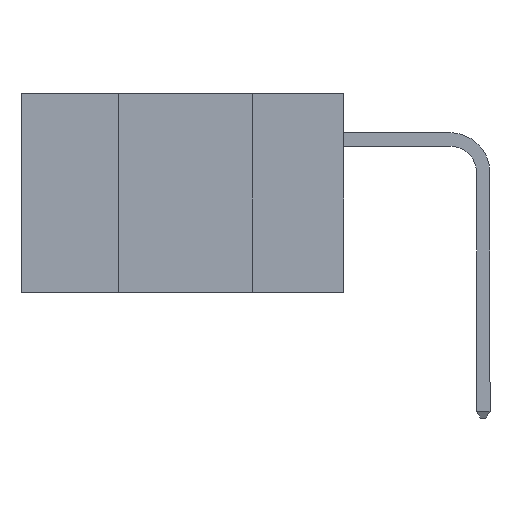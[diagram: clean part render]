
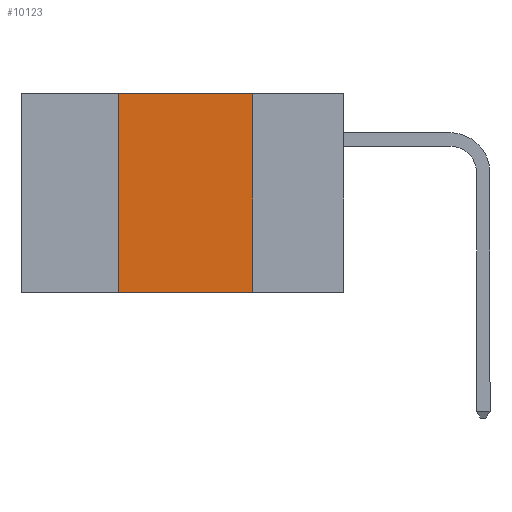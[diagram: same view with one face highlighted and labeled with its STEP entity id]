
A CAD part, left-side view. The second image highlights one B-rep face of the part: STEP entity #10123.
In plain terms, the highlighted planar face has unit normal (-1, 0, 0).
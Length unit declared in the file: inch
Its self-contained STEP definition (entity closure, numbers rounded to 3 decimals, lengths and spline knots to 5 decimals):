
#3 = VECTOR ( 'NONE', #8634, 39.37008 ) ;
#94 = VECTOR ( 'NONE', #7449, 39.37008 ) ;
#901 = CARTESIAN_POINT ( 'NONE',  ( 0., 0.42, -0.37 ) ) ;
#1397 = ORIENTED_EDGE ( 'NONE', *, *, #11086, .F. ) ;
#2379 = FACE_OUTER_BOUND ( 'NONE', #9345, .T. ) ;
#2935 = CARTESIAN_POINT ( 'NONE',  ( 0., 0.17, 0. ) ) ;
#3398 = DIRECTION ( 'NONE',  ( 0., 0., 1. ) ) ;
#3861 = ORIENTED_EDGE ( 'NONE', *, *, #10646, .F. ) ;
#4122 = DIRECTION ( 'NONE',  ( 1., 0., 0. ) ) ;
#6279 = CARTESIAN_POINT ( 'NONE',  ( 0., 0.42, 0. ) ) ;
#6546 = VERTEX_POINT ( 'NONE', #17685 ) ;
#6802 = LINE ( 'NONE', #18522, #3 ) ;
#7359 = VECTOR ( 'NONE', #3398, 39.37008 ) ;
#7449 = DIRECTION ( 'NONE',  ( 0., 0., -1. ) ) ;
#7548 = DIRECTION ( 'NONE',  ( 0., -1., 0. ) ) ;
#7819 = LINE ( 'NONE', #6279, #7359 ) ;
#8634 = DIRECTION ( 'NONE',  ( 0., -1., 0. ) ) ;
#8967 = CARTESIAN_POINT ( 'NONE',  ( 0., 0.6, 0. ) ) ;
#9027 = EDGE_CURVE ( 'NONE', #12057, #12809, #14076, .T. ) ;
#9345 = EDGE_LOOP ( 'NONE', ( #1397, #15475, #3861, #18478 ) ) ;
#9872 = CARTESIAN_POINT ( 'NONE',  ( 0., 0.42, 0. ) ) ;
#9939 = PLANE ( 'NONE',  #12224 ) ;
#10123 = ADVANCED_FACE ( 'NONE', ( #2379 ), #9939, .F. ) ;
#10377 = VECTOR ( 'NONE', #7548, 39.37008 ) ;
#10646 = EDGE_CURVE ( 'NONE', #13736, #12057, #7819, .T. ) ;
#11086 = EDGE_CURVE ( 'NONE', #12809, #6546, #11169, .T. ) ;
#11169 = LINE ( 'NONE', #13118, #94 ) ;
#12057 = VERTEX_POINT ( 'NONE', #9872 ) ;
#12224 = AXIS2_PLACEMENT_3D ( 'NONE', #12736, #4122, #14140 ) ;
#12736 = CARTESIAN_POINT ( 'NONE',  ( 0., 0.6, 0. ) ) ;
#12809 = VERTEX_POINT ( 'NONE', #2935 ) ;
#13118 = CARTESIAN_POINT ( 'NONE',  ( 0., 0.17, 0. ) ) ;
#13736 = VERTEX_POINT ( 'NONE', #901 ) ;
#14076 = LINE ( 'NONE', #8967, #10377 ) ;
#14140 = DIRECTION ( 'NONE',  ( 0., 0., -1. ) ) ;
#15475 = ORIENTED_EDGE ( 'NONE', *, *, #9027, .F. ) ;
#15847 = EDGE_CURVE ( 'NONE', #13736, #6546, #6802, .T. ) ;
#17685 = CARTESIAN_POINT ( 'NONE',  ( 0., 0.17, -0.37 ) ) ;
#18478 = ORIENTED_EDGE ( 'NONE', *, *, #15847, .T. ) ;
#18522 = CARTESIAN_POINT ( 'NONE',  ( 0., 0.6, -0.37 ) ) ;
